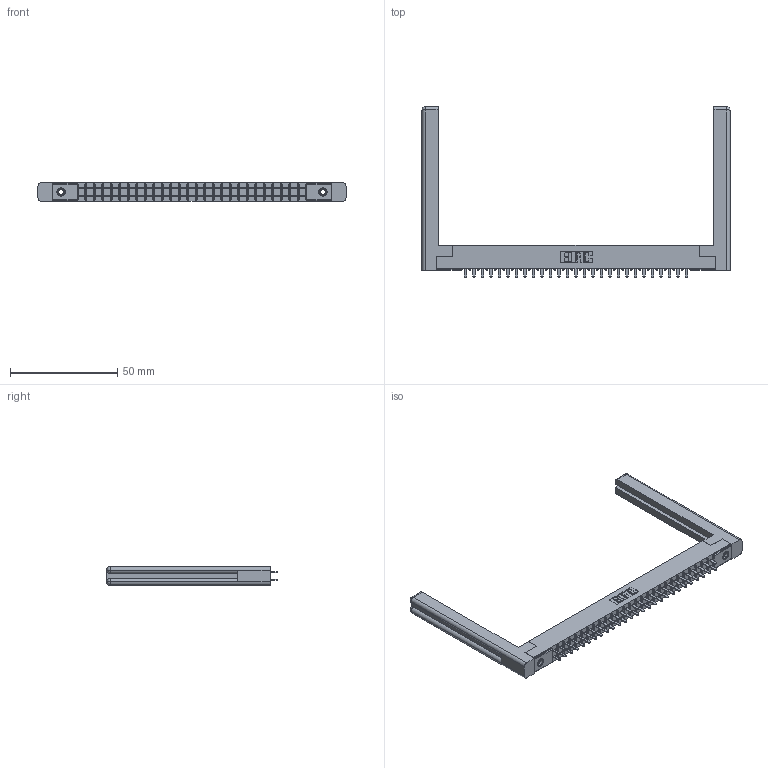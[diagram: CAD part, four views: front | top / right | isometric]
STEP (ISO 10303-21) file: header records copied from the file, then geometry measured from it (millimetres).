
FILE_DESCRIPTION (( 'STEP AP203' ), '1' );
FILE_NAME ('355-054-521-258.STEP', '2019-09-11T17:04:46', ( '' ), ( '' ), 'SwSTEP 2.0', 'SolidWorks 2016', '' );
FILE_SCHEMA (( 'CONFIG_CONTROL_DESIGN' ));
Length unit declared in the file: inch
Products named in the file (5): 345-250-001_345-250-001-102; 305-290-001_521; 355-054-521-258; 307-220-058; 305 Part_.156 Dia
Assembly tree (59 placements, depth 2):
  355-054-521-258
    305 Part_.156 Dia
    305-290-001_521  x54
    345-250-001_345-250-001-102  x2
    307-220-058  x2
Bounding box: 143.61 x 79.5 x 8.71 mm (x, y, z)
Volume: 16668.4 mm3; surface area: 22018.5 mm2
Topology: 59 solids, 59 shells, 2742 faces, 7771 edges, 5022 vertices
Faces by surface type: plane 1610, cylinder 1000, sphere 108, cone 12, torus 12
Entity records: 33573 total; most frequent: CARTESIAN_POINT 5570, ORIENTED_EDGE 5468, DIRECTION 5362, EDGE_CURVE 2734, LINE 2186, VECTOR 2186, VERTEX_POINT 1742, AXIS2_PLACEMENT_3D 1588
